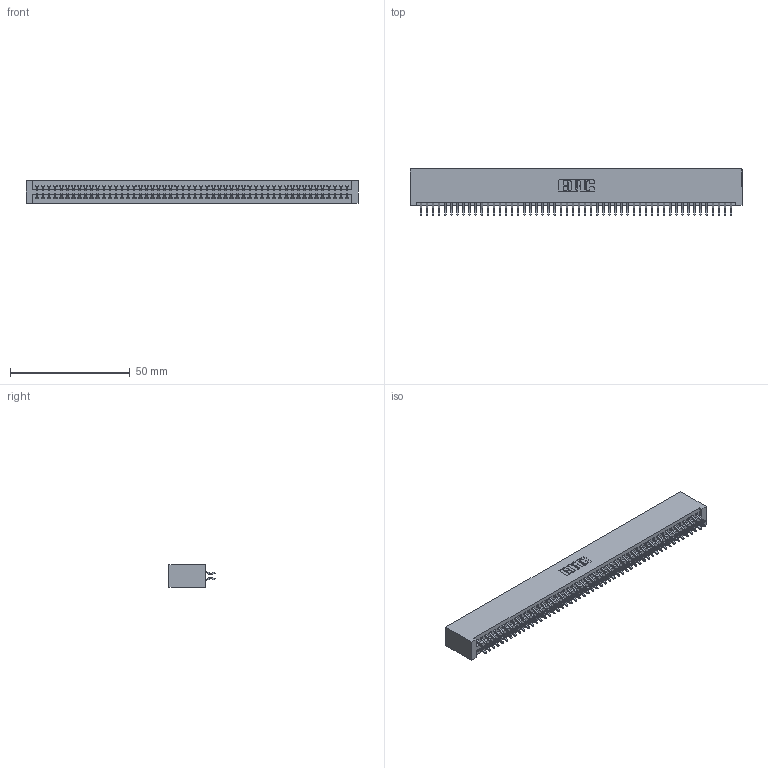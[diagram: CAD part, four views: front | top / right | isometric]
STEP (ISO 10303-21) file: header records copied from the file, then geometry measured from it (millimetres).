
FILE_DESCRIPTION (( 'STEP AP203' ), '1' );
FILE_NAME ('345-104-556-201.STEP', '2019-11-03T12:46:52', ( '' ), ( '' ), 'SwSTEP 2.0', 'SolidWorks 2016', '' );
FILE_SCHEMA (( 'CONFIG_CONTROL_DESIGN' ));
Length unit declared in the file: inch
Products named in the file (3): 345-292-001_556 Tail; 345-104-556-201; 345 Part_No Mounting Lugs
Assembly tree (105 placements, depth 2):
  345-104-556-201
    345 Part_No Mounting Lugs
    345-292-001_556 Tail  x104
Bounding box: 138.68 x 19.24 x 9.4 mm (x, y, z)
Volume: 14176.5 mm3; surface area: 21361.2 mm2
Topology: 105 solids, 105 shells, 5942 faces, 17685 edges, 11650 vertices
Faces by surface type: plane 3924, cylinder 2018
Entity records: 39397 total; most frequent: CARTESIAN_POINT 6608, ORIENTED_EDGE 6530, DIRECTION 5797, EDGE_CURVE 3265, LINE 2925, VECTOR 2925, VERTEX_POINT 2174, AXIS2_PLACEMENT_3D 1436
